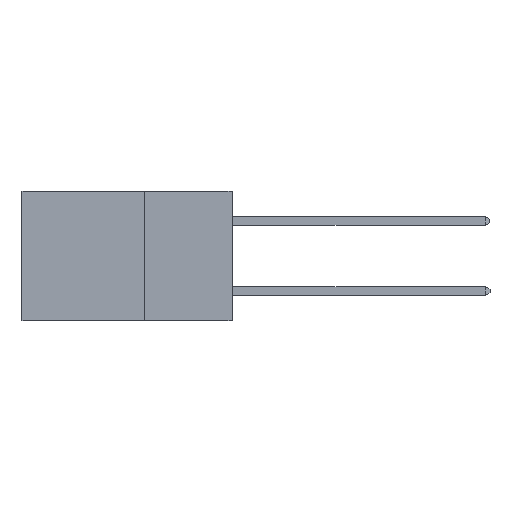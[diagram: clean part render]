
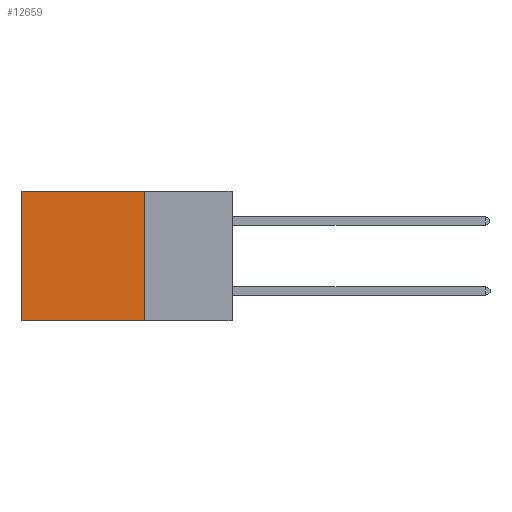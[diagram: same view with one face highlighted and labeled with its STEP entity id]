
A CAD part, left-side view. The second image highlights one B-rep face of the part: STEP entity #12659.
In plain terms, the highlighted planar face has unit normal (-1, 0, 0).
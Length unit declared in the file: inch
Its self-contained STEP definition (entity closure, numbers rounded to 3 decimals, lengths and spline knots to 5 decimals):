
#89 = EDGE_CURVE ( 'NONE', #17735, #176, #11707, .T. ) ;
#176 = VERTEX_POINT ( 'NONE', #14810 ) ;
#1832 = CARTESIAN_POINT ( 'NONE',  ( 0.2875, 0.25, 0. ) ) ;
#3104 = ORIENTED_EDGE ( 'NONE', *, *, #89, .F. ) ;
#4039 = PLANE ( 'NONE',  #20770 ) ;
#4188 = DIRECTION ( 'NONE',  ( 1., 0., 0. ) ) ;
#4204 = EDGE_LOOP ( 'NONE', ( #6358, #3104, #22572, #4238 ) ) ;
#4238 = ORIENTED_EDGE ( 'NONE', *, *, #11735, .T. ) ;
#4556 = FACE_OUTER_BOUND ( 'NONE', #4204, .T. ) ;
#4970 = VECTOR ( 'NONE', #12271, 39.37008 ) ;
#4984 = VERTEX_POINT ( 'NONE', #22534 ) ;
#5403 = LINE ( 'NONE', #16835, #9454 ) ;
#5588 = DIRECTION ( 'NONE',  ( 0., 1., 0. ) ) ;
#6358 = ORIENTED_EDGE ( 'NONE', *, *, #9902, .T. ) ;
#9454 = VECTOR ( 'NONE', #9810, 39.37008 ) ;
#9810 = DIRECTION ( 'NONE',  ( 0., 0., -1. ) ) ;
#9902 = EDGE_CURVE ( 'NONE', #10527, #176, #14876, .T. ) ;
#10527 = VERTEX_POINT ( 'NONE', #14354 ) ;
#11178 = VECTOR ( 'NONE', #17667, 39.37008 ) ;
#11707 = LINE ( 'NONE', #17521, #11178 ) ;
#11735 = EDGE_CURVE ( 'NONE', #4984, #10527, #14505, .T. ) ;
#12049 = EDGE_CURVE ( 'NONE', #4984, #17735, #5403, .T. ) ;
#12271 = DIRECTION ( 'NONE',  ( 0., 0., -1. ) ) ;
#12659 = ADVANCED_FACE ( 'NONE', ( #4556 ), #4039, .F. ) ;
#14354 = CARTESIAN_POINT ( 'NONE',  ( 0.2875, 0.6, 0. ) ) ;
#14505 = LINE ( 'NONE', #1832, #19092 ) ;
#14653 = CARTESIAN_POINT ( 'NONE',  ( 0.2875, 0.25, -0.37 ) ) ;
#14810 = CARTESIAN_POINT ( 'NONE',  ( 0.2875, 0.6, -0.37 ) ) ;
#14876 = LINE ( 'NONE', #20844, #4970 ) ;
#16496 = DIRECTION ( 'NONE',  ( 0., 0., -1. ) ) ;
#16835 = CARTESIAN_POINT ( 'NONE',  ( 0.2875, 0.25, 0. ) ) ;
#17521 = CARTESIAN_POINT ( 'NONE',  ( 0.2875, 0.25, -0.37 ) ) ;
#17667 = DIRECTION ( 'NONE',  ( 0., 1., 0. ) ) ;
#17735 = VERTEX_POINT ( 'NONE', #14653 ) ;
#19092 = VECTOR ( 'NONE', #5588, 39.37008 ) ;
#19890 = CARTESIAN_POINT ( 'NONE',  ( 0.2875, 0.25, 0. ) ) ;
#20770 = AXIS2_PLACEMENT_3D ( 'NONE', #19890, #4188, #16496 ) ;
#20844 = CARTESIAN_POINT ( 'NONE',  ( 0.2875, 0.6, 0. ) ) ;
#22534 = CARTESIAN_POINT ( 'NONE',  ( 0.2875, 0.25, 0. ) ) ;
#22572 = ORIENTED_EDGE ( 'NONE', *, *, #12049, .F. ) ;
